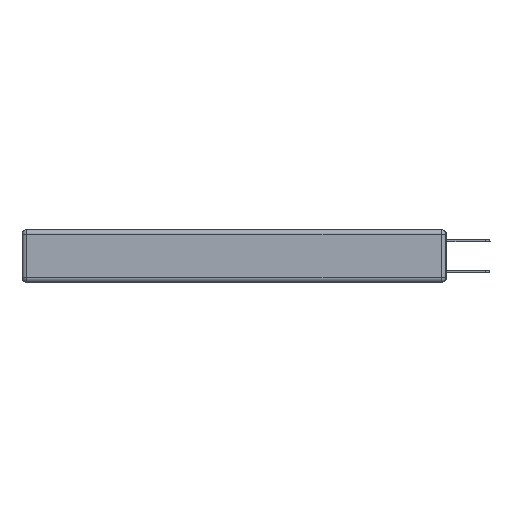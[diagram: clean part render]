
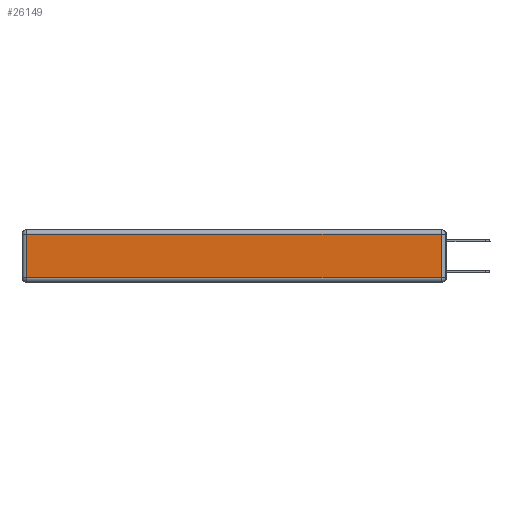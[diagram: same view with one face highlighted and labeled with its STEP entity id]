
A CAD part, left-side view. The second image highlights one B-rep face of the part: STEP entity #26149.
In plain terms, the highlighted planar face has unit normal (-1, 0, 0).
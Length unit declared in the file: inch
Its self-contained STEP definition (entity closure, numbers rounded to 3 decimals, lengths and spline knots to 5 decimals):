
#23 = DIRECTION ( 'NONE',  ( 0., 0., 1. ) ) ;
#1163 = ORIENTED_EDGE ( 'NONE', *, *, #12999, .T. ) ;
#1468 = VERTEX_POINT ( 'NONE', #22291 ) ;
#2278 = VECTOR ( 'NONE', #23, 39.37008 ) ;
#3439 = ORIENTED_EDGE ( 'NONE', *, *, #20928, .T. ) ;
#3462 = DIRECTION ( 'NONE',  ( 0., 0., -1. ) ) ;
#5657 = PLANE ( 'NONE',  #26680 ) ;
#6886 = VERTEX_POINT ( 'NONE', #9981 ) ;
#7836 = DIRECTION ( 'NONE',  ( 0., -1., 0. ) ) ;
#7866 = CARTESIAN_POINT ( 'NONE',  ( 0., 0., -0.343 ) ) ;
#8394 = FACE_OUTER_BOUND ( 'NONE', #25560, .T. ) ;
#8922 = LINE ( 'NONE', #12382, #11861 ) ;
#9981 = CARTESIAN_POINT ( 'NONE',  ( 0., 0.03, -0.313 ) ) ;
#11011 = LINE ( 'NONE', #20623, #19190 ) ;
#11861 = VECTOR ( 'NONE', #7836, 39.37008 ) ;
#12382 = CARTESIAN_POINT ( 'NONE',  ( 0., 0., -0.313 ) ) ;
#12857 = CARTESIAN_POINT ( 'NONE',  ( 0., 2.72, -0.03 ) ) ;
#12934 = LINE ( 'NONE', #18200, #20120 ) ;
#12999 = EDGE_CURVE ( 'NONE', #24205, #24840, #12934, .T. ) ;
#15781 = ORIENTED_EDGE ( 'NONE', *, *, #19678, .T. ) ;
#17190 = ORIENTED_EDGE ( 'NONE', *, *, #26227, .T. ) ;
#17379 = LINE ( 'NONE', #22884, #2278 ) ;
#18200 = CARTESIAN_POINT ( 'NONE',  ( 0., 2.72, -0.343 ) ) ;
#19190 = VECTOR ( 'NONE', #26984, 39.37008 ) ;
#19678 = EDGE_CURVE ( 'NONE', #24840, #6886, #8922, .T. ) ;
#20120 = VECTOR ( 'NONE', #3462, 39.37008 ) ;
#20623 = CARTESIAN_POINT ( 'NONE',  ( 0., 2.75, -0.03 ) ) ;
#20928 = EDGE_CURVE ( 'NONE', #6886, #1468, #17379, .T. ) ;
#22291 = CARTESIAN_POINT ( 'NONE',  ( 0., 0.03, -0.03 ) ) ;
#22798 = DIRECTION ( 'NONE',  ( 0., 0., 1. ) ) ;
#22884 = CARTESIAN_POINT ( 'NONE',  ( 0., 0.03, -0.343 ) ) ;
#23577 = CARTESIAN_POINT ( 'NONE',  ( 0., 2.72, -0.313 ) ) ;
#24205 = VERTEX_POINT ( 'NONE', #12857 ) ;
#24840 = VERTEX_POINT ( 'NONE', #23577 ) ;
#25560 = EDGE_LOOP ( 'NONE', ( #15781, #3439, #17190, #1163 ) ) ;
#26149 = ADVANCED_FACE ( 'NONE', ( #8394 ), #5657, .T. ) ;
#26227 = EDGE_CURVE ( 'NONE', #1468, #24205, #11011, .T. ) ;
#26625 = DIRECTION ( 'NONE',  ( -1., 0., 0. ) ) ;
#26680 = AXIS2_PLACEMENT_3D ( 'NONE', #7866, #26625, #22798 ) ;
#26984 = DIRECTION ( 'NONE',  ( 0., 1., 0. ) ) ;
